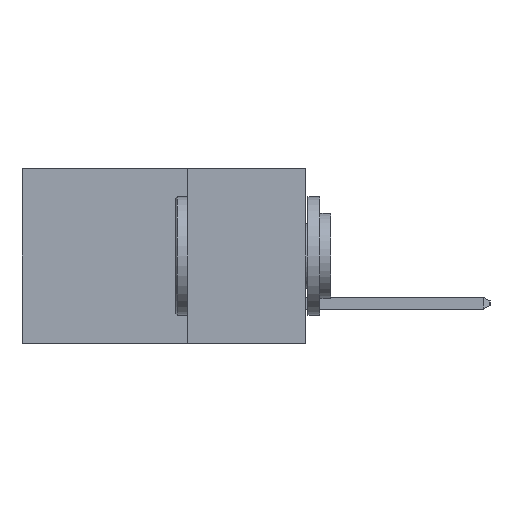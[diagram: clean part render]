
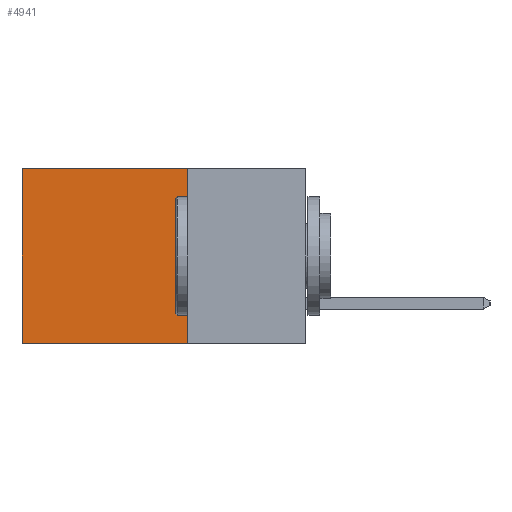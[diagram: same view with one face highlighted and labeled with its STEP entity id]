
A CAD part, left-side view. The second image highlights one B-rep face of the part: STEP entity #4941.
In plain terms, the highlighted planar face has unit normal (-1, 0, 0).
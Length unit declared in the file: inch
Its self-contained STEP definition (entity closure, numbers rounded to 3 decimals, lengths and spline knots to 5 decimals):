
#89 = EDGE_CURVE ( 'NONE', #5411, #1932, #17009, .T. ) ;
#930 = AXIS2_PLACEMENT_3D ( 'NONE', #9989, #1518, #16879 ) ;
#999 = EDGE_CURVE ( 'NONE', #1932, #13374, #12658, .T. ) ;
#1518 = DIRECTION ( 'NONE',  ( 1., 0., 0. ) ) ;
#1842 = DIRECTION ( 'NONE',  ( 0., 1., 0. ) ) ;
#1932 = VERTEX_POINT ( 'NONE', #9927 ) ;
#1996 = LINE ( 'NONE', #7670, #9443 ) ;
#2174 = DIRECTION ( 'NONE',  ( 0., 0., -1. ) ) ;
#4366 = ORIENTED_EDGE ( 'NONE', *, *, #14084, .T. ) ;
#4897 = ORIENTED_EDGE ( 'NONE', *, *, #89, .F. ) ;
#4941 = ADVANCED_FACE ( 'NONE', ( #12087 ), #6944, .F. ) ;
#5411 = VERTEX_POINT ( 'NONE', #13742 ) ;
#6944 = PLANE ( 'NONE',  #930 ) ;
#7670 = CARTESIAN_POINT ( 'NONE',  ( 0.298, 0.25, 0. ) ) ;
#8474 = ORIENTED_EDGE ( 'NONE', *, *, #999, .F. ) ;
#8621 = VECTOR ( 'NONE', #14971, 39.37008 ) ;
#9023 = VECTOR ( 'NONE', #12272, 39.37008 ) ;
#9246 = VECTOR ( 'NONE', #2174, 39.37008 ) ;
#9443 = VECTOR ( 'NONE', #1842, 39.37008 ) ;
#9927 = CARTESIAN_POINT ( 'NONE',  ( 0.298, 0.25, -0.37 ) ) ;
#9989 = CARTESIAN_POINT ( 'NONE',  ( 0.298, 0.25, 0. ) ) ;
#10887 = CARTESIAN_POINT ( 'NONE',  ( 0.298, 0.6, 0. ) ) ;
#11437 = EDGE_LOOP ( 'NONE', ( #4366, #8474, #4897, #16007 ) ) ;
#11850 = CARTESIAN_POINT ( 'NONE',  ( 0.298, 0.25, 0. ) ) ;
#11972 = CARTESIAN_POINT ( 'NONE',  ( 0.298, 0.25, -0.37 ) ) ;
#12087 = FACE_OUTER_BOUND ( 'NONE', #11437, .T. ) ;
#12272 = DIRECTION ( 'NONE',  ( 0., 1., 0. ) ) ;
#12658 = LINE ( 'NONE', #11972, #9023 ) ;
#12713 = CARTESIAN_POINT ( 'NONE',  ( 0.298, 0.6, -0.37 ) ) ;
#13374 = VERTEX_POINT ( 'NONE', #12713 ) ;
#13742 = CARTESIAN_POINT ( 'NONE',  ( 0.298, 0.25, 0. ) ) ;
#13849 = EDGE_CURVE ( 'NONE', #5411, #16109, #1996, .T. ) ;
#14084 = EDGE_CURVE ( 'NONE', #16109, #13374, #15928, .T. ) ;
#14843 = CARTESIAN_POINT ( 'NONE',  ( 0.298, 0.6, 0. ) ) ;
#14971 = DIRECTION ( 'NONE',  ( 0., 0., -1. ) ) ;
#15928 = LINE ( 'NONE', #10887, #8621 ) ;
#16007 = ORIENTED_EDGE ( 'NONE', *, *, #13849, .T. ) ;
#16109 = VERTEX_POINT ( 'NONE', #14843 ) ;
#16879 = DIRECTION ( 'NONE',  ( 0., 0., -1. ) ) ;
#17009 = LINE ( 'NONE', #11850, #9246 ) ;
